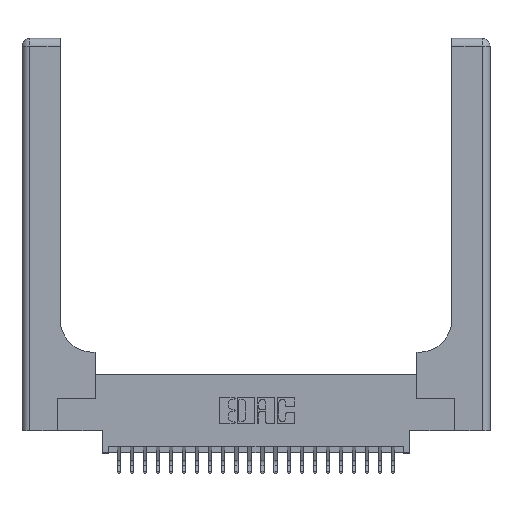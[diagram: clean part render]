
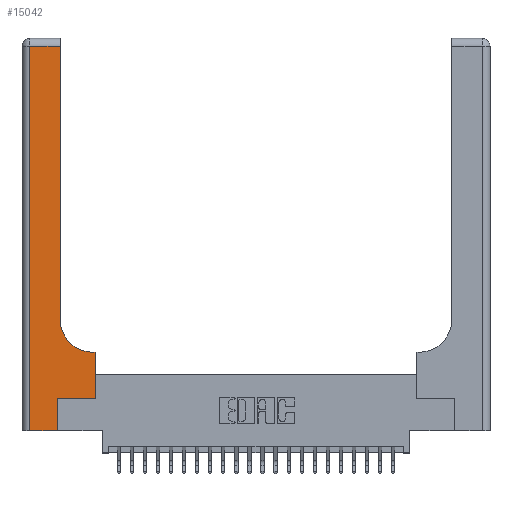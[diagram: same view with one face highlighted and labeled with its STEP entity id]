
A CAD part, top view. The second image highlights one B-rep face of the part: STEP entity #15042.
In plain terms, the highlighted planar face has unit normal (0, 0, 1).
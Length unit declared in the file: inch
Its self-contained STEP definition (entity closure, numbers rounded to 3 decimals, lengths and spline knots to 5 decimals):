
#148 = VECTOR ( 'NONE', #22140, 39.37008 ) ;
#287 = EDGE_CURVE ( 'NONE', #18885, #3327, #5023, .T. ) ;
#592 = LINE ( 'NONE', #18111, #7059 ) ;
#635 = CARTESIAN_POINT ( 'NONE',  ( 0.2915, 2.94, 0.37 ) ) ;
#889 = CARTESIAN_POINT ( 'NONE',  ( 0.5415, 0.85, 0.37 ) ) ;
#1256 = CARTESIAN_POINT ( 'NONE',  ( 0.06, 0., 0.37 ) ) ;
#1591 = ORIENTED_EDGE ( 'NONE', *, *, #20575, .T. ) ;
#1683 = LINE ( 'NONE', #1962, #148 ) ;
#1868 = LINE ( 'NONE', #15914, #22521 ) ;
#1962 = CARTESIAN_POINT ( 'NONE',  ( 0.2915, 3., 0.37 ) ) ;
#2140 = VECTOR ( 'NONE', #13978, 39.37008 ) ;
#2304 = LINE ( 'NONE', #5766, #9674 ) ;
#3327 = VERTEX_POINT ( 'NONE', #24110 ) ;
#3341 = DIRECTION ( 'NONE',  ( 0., 0., -1. ) ) ;
#3475 = DIRECTION ( 'NONE',  ( -1., 0., 0. ) ) ;
#4325 = AXIS2_PLACEMENT_3D ( 'NONE', #19263, #3341, #17178 ) ;
#4353 = CARTESIAN_POINT ( 'NONE',  ( 0.269, 0., 0.37 ) ) ;
#5023 = LINE ( 'NONE', #24095, #7484 ) ;
#5029 = EDGE_CURVE ( 'NONE', #24193, #16476, #1683, .T. ) ;
#5120 = DIRECTION ( 'NONE',  ( 0., -1., 0. ) ) ;
#5158 = EDGE_CURVE ( 'NONE', #10148, #21451, #11514, .T. ) ;
#5202 = AXIS2_PLACEMENT_3D ( 'NONE', #889, #8863, #10924 ) ;
#5215 = ORIENTED_EDGE ( 'NONE', *, *, #5158, .T. ) ;
#5353 = CARTESIAN_POINT ( 'NONE',  ( 0.269, 0.25, 0.37 ) ) ;
#5400 = DIRECTION ( 'NONE',  ( 1., 0., 0. ) ) ;
#5766 = CARTESIAN_POINT ( 'NONE',  ( 0., 2.94, 0.37 ) ) ;
#5770 = CIRCLE ( 'NONE', #5202, 0.25 ) ;
#7059 = VECTOR ( 'NONE', #5120, 39.37008 ) ;
#7484 = VECTOR ( 'NONE', #18383, 39.37008 ) ;
#8590 = FACE_OUTER_BOUND ( 'NONE', #14913, .T. ) ;
#8654 = EDGE_CURVE ( 'NONE', #16476, #23519, #2304, .T. ) ;
#8863 = DIRECTION ( 'NONE',  ( 0., 0., -1. ) ) ;
#9006 = VECTOR ( 'NONE', #5400, 39.37008 ) ;
#9302 = CARTESIAN_POINT ( 'NONE',  ( 0.5585, 0.25, 0.37 ) ) ;
#9430 = CARTESIAN_POINT ( 'NONE',  ( 0.269, 0.25, 0.37 ) ) ;
#9490 = ORIENTED_EDGE ( 'NONE', *, *, #12975, .T. ) ;
#9674 = VECTOR ( 'NONE', #3475, 39.37008 ) ;
#10148 = VERTEX_POINT ( 'NONE', #4353 ) ;
#10264 = CARTESIAN_POINT ( 'NONE',  ( 0.2915, 0.85, 0.37 ) ) ;
#10924 = DIRECTION ( 'NONE',  ( 1., 0., 0. ) ) ;
#11514 = LINE ( 'NONE', #22023, #15225 ) ;
#11583 = ORIENTED_EDGE ( 'NONE', *, *, #287, .T. ) ;
#11912 = CARTESIAN_POINT ( 'NONE',  ( 0.5585, 0.25, 0.37 ) ) ;
#12975 = EDGE_CURVE ( 'NONE', #23519, #21439, #592, .T. ) ;
#13978 = DIRECTION ( 'NONE',  ( 0., 1., 0. ) ) ;
#14219 = LINE ( 'NONE', #9430, #9006 ) ;
#14913 = EDGE_LOOP ( 'NONE', ( #20509, #19170, #9490, #15387, #5215, #24746, #1591, #11583, #16191 ) ) ;
#15042 = ADVANCED_FACE ( 'NONE', ( #8590 ), #17092, .F. ) ;
#15225 = VECTOR ( 'NONE', #24033, 39.37008 ) ;
#15387 = ORIENTED_EDGE ( 'NONE', *, *, #16255, .T. ) ;
#15914 = CARTESIAN_POINT ( 'NONE',  ( 0., 0., 0.37 ) ) ;
#16191 = ORIENTED_EDGE ( 'NONE', *, *, #17450, .T. ) ;
#16255 = EDGE_CURVE ( 'NONE', #21439, #10148, #1868, .T. ) ;
#16476 = VERTEX_POINT ( 'NONE', #635 ) ;
#17092 = PLANE ( 'NONE',  #4325 ) ;
#17178 = DIRECTION ( 'NONE',  ( -1., 0., 0. ) ) ;
#17222 = LINE ( 'NONE', #11912, #2140 ) ;
#17450 = EDGE_CURVE ( 'NONE', #3327, #24193, #5770, .T. ) ;
#18111 = CARTESIAN_POINT ( 'NONE',  ( 0.06, 3., 0.37 ) ) ;
#18383 = DIRECTION ( 'NONE',  ( -1., 0., 0. ) ) ;
#18885 = VERTEX_POINT ( 'NONE', #21400 ) ;
#19170 = ORIENTED_EDGE ( 'NONE', *, *, #8654, .T. ) ;
#19263 = CARTESIAN_POINT ( 'NONE',  ( 0., 3., 0.37 ) ) ;
#19729 = VERTEX_POINT ( 'NONE', #9302 ) ;
#20509 = ORIENTED_EDGE ( 'NONE', *, *, #5029, .T. ) ;
#20575 = EDGE_CURVE ( 'NONE', #19729, #18885, #17222, .T. ) ;
#21400 = CARTESIAN_POINT ( 'NONE',  ( 0.5585, 0.6, 0.37 ) ) ;
#21439 = VERTEX_POINT ( 'NONE', #1256 ) ;
#21451 = VERTEX_POINT ( 'NONE', #5353 ) ;
#22023 = CARTESIAN_POINT ( 'NONE',  ( 0.269, 0., 0.37 ) ) ;
#22140 = DIRECTION ( 'NONE',  ( 0., 1., 0. ) ) ;
#22521 = VECTOR ( 'NONE', #24124, 39.37008 ) ;
#23519 = VERTEX_POINT ( 'NONE', #24144 ) ;
#24033 = DIRECTION ( 'NONE',  ( 0., 1., 0. ) ) ;
#24095 = CARTESIAN_POINT ( 'NONE',  ( 0.2915, 0.6, 0.37 ) ) ;
#24110 = CARTESIAN_POINT ( 'NONE',  ( 0.5415, 0.6, 0.37 ) ) ;
#24124 = DIRECTION ( 'NONE',  ( 1., 0., 0. ) ) ;
#24144 = CARTESIAN_POINT ( 'NONE',  ( 0.06, 2.94, 0.37 ) ) ;
#24193 = VERTEX_POINT ( 'NONE', #10264 ) ;
#24484 = EDGE_CURVE ( 'NONE', #21451, #19729, #14219, .T. ) ;
#24746 = ORIENTED_EDGE ( 'NONE', *, *, #24484, .T. ) ;
